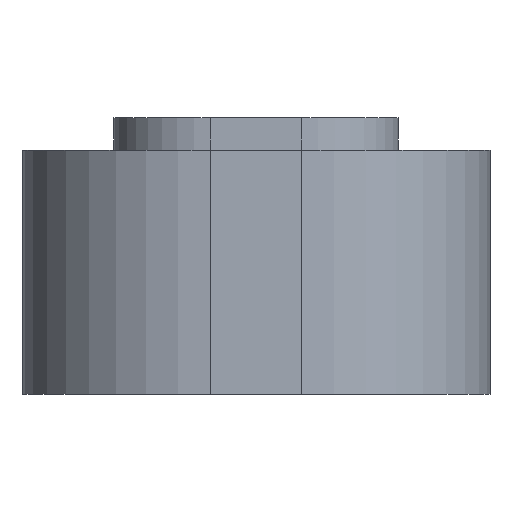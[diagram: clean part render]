
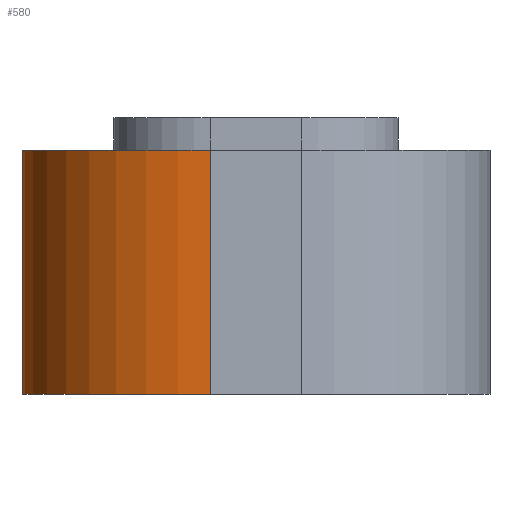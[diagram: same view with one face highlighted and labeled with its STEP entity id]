
A CAD part, front view. The second image highlights one B-rep face of the part: STEP entity #580.
In plain terms, the highlighted cylindrical face has radius 4.63 mm (diameter 9.26 mm), a partial arc.
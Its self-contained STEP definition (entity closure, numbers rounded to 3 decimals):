
#25=CIRCLE('',#631,4.63);
#26=CIRCLE('',#632,4.63);
#56=CYLINDRICAL_SURFACE('',#630,4.63);
#74=FACE_OUTER_BOUND('',#108,.T.);
#108=EDGE_LOOP('',(#403,#404,#405,#406));
#154=LINE('',#898,#206);
#155=LINE('',#904,#207);
#206=VECTOR('',#710,10.);
#207=VECTOR('',#717,10.);
#257=VERTEX_POINT('',#894);
#258=VERTEX_POINT('',#896);
#259=VERTEX_POINT('',#900);
#260=VERTEX_POINT('',#902);
#316=EDGE_CURVE('',#257,#258,#154,.T.);
#317=EDGE_CURVE('',#257,#259,#25,.T.);
#318=EDGE_CURVE('',#260,#258,#26,.T.);
#319=EDGE_CURVE('',#259,#260,#155,.T.);
#403=ORIENTED_EDGE('',*,*,#317,.F.);
#404=ORIENTED_EDGE('',*,*,#316,.T.);
#405=ORIENTED_EDGE('',*,*,#318,.F.);
#406=ORIENTED_EDGE('',*,*,#319,.F.);
#580=ADVANCED_FACE('',(#74),#56,.T.);
#630=AXIS2_PLACEMENT_3D('',#899,#711,#712);
#631=AXIS2_PLACEMENT_3D('',#901,#713,#714);
#632=AXIS2_PLACEMENT_3D('',#903,#715,#716);
#710=DIRECTION('',(0.,0.,-1.));
#711=DIRECTION('center_axis',(0.,0.,-1.));
#712=DIRECTION('ref_axis',(-1.,0.,0.));
#713=DIRECTION('center_axis',(0.,0.,1.));
#714=DIRECTION('ref_axis',(-1.,0.,0.));
#715=DIRECTION('center_axis',(0.,0.,-1.));
#716=DIRECTION('ref_axis',(-1.,0.,0.));
#717=DIRECTION('',(0.,0.,-1.));
#894=CARTESIAN_POINT('',(-5.75,10.38,-0.8));
#896=CARTESIAN_POINT('',(-5.75,10.38,-6.8));
#898=CARTESIAN_POINT('',(-5.75,10.38,-0.8));
#899=CARTESIAN_POINT('Origin',(-1.12,10.38,-0.8));
#900=CARTESIAN_POINT('',(-1.12,5.75,-0.8));
#901=CARTESIAN_POINT('Origin',(-1.12,10.38,-0.8));
#902=CARTESIAN_POINT('',(-1.12,5.75,-6.8));
#903=CARTESIAN_POINT('Origin',(-1.12,10.38,-6.8));
#904=CARTESIAN_POINT('',(-1.12,5.75,-0.8));
